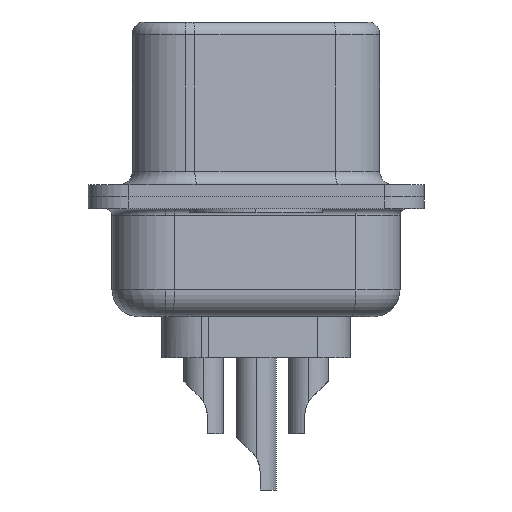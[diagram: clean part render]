
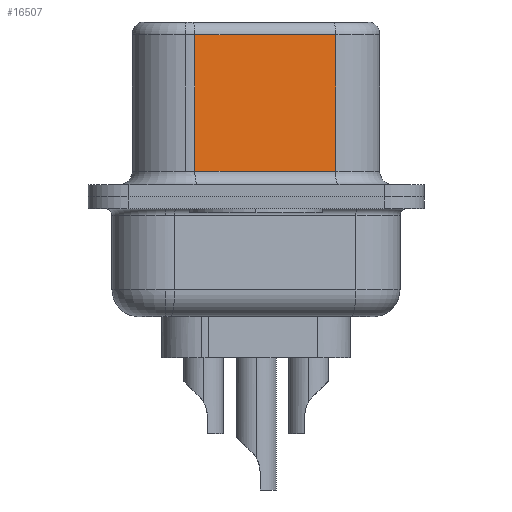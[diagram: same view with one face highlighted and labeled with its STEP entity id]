
A CAD part, left-side view. The second image highlights one B-rep face of the part: STEP entity #16507.
In plain terms, the highlighted planar face has unit normal (-0.985, -0.174, 0).
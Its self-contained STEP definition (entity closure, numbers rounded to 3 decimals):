
#114 = DIRECTION ( 'NONE',  ( 0.985, 0.174, 0. ) ) ;
#605 = AXIS2_PLACEMENT_3D ( 'NONE', #13615, #114, #6886 ) ;
#1088 = ORIENTED_EDGE ( 'NONE', *, *, #12718, .T. ) ;
#1789 = VERTEX_POINT ( 'NONE', #17715 ) ;
#2067 = LINE ( 'NONE', #8825, #8016 ) ;
#2081 = EDGE_CURVE ( 'NONE', #20152, #1789, #10763, .T. ) ;
#2378 = CARTESIAN_POINT ( 'NONE',  ( 4.546, -2.987, 0.95 ) ) ;
#2436 = ORIENTED_EDGE ( 'NONE', *, *, #13427, .F. ) ;
#3622 = DIRECTION ( 'NONE',  ( 0., 0., -1. ) ) ;
#3859 = ORIENTED_EDGE ( 'NONE', *, *, #2081, .T. ) ;
#4138 = CARTESIAN_POINT ( 'NONE',  ( 4.546, -2.987, 6.07 ) ) ;
#4976 = CARTESIAN_POINT ( 'NONE',  ( 4.546, -2.987, 0.95 ) ) ;
#5349 = DIRECTION ( 'NONE',  ( -0.174, 0.985, 0. ) ) ;
#5482 = DIRECTION ( 'NONE',  ( 0., 0., -1. ) ) ;
#6273 = VERTEX_POINT ( 'NONE', #13761 ) ;
#6886 = DIRECTION ( 'NONE',  ( -0.174, 0.985, 0. ) ) ;
#7346 = CARTESIAN_POINT ( 'NONE',  ( 4.546, -2.987, 6.07 ) ) ;
#8016 = VECTOR ( 'NONE', #3622, 1000. ) ;
#8825 = CARTESIAN_POINT ( 'NONE',  ( 3.615, 2.293, 6.57 ) ) ;
#9339 = CARTESIAN_POINT ( 'NONE',  ( 4.546, -2.987, 6.57 ) ) ;
#9367 = EDGE_LOOP ( 'NONE', ( #2436, #3859, #1088, #20185 ) ) ;
#10199 = FACE_OUTER_BOUND ( 'NONE', #9367, .T. ) ;
#10763 = LINE ( 'NONE', #7346, #10787 ) ;
#10787 = VECTOR ( 'NONE', #5349, 1000. ) ;
#10822 = DIRECTION ( 'NONE',  ( 0.174, -0.985, 0. ) ) ;
#12718 = EDGE_CURVE ( 'NONE', #1789, #6273, #2067, .T. ) ;
#13427 = EDGE_CURVE ( 'NONE', #20152, #19004, #21044, .T. ) ;
#13615 = CARTESIAN_POINT ( 'NONE',  ( 4.546, -2.987, 6.57 ) ) ;
#13761 = CARTESIAN_POINT ( 'NONE',  ( 3.615, 2.293, 0.95 ) ) ;
#16497 = VECTOR ( 'NONE', #10822, 1000. ) ;
#16507 = ADVANCED_FACE ( 'NONE', ( #10199 ), #20249, .F. ) ;
#17049 = EDGE_CURVE ( 'NONE', #6273, #19004, #20120, .T. ) ;
#17715 = CARTESIAN_POINT ( 'NONE',  ( 3.615, 2.293, 6.07 ) ) ;
#18142 = VECTOR ( 'NONE', #5482, 1000. ) ;
#19004 = VERTEX_POINT ( 'NONE', #2378 ) ;
#20120 = LINE ( 'NONE', #4976, #16497 ) ;
#20152 = VERTEX_POINT ( 'NONE', #4138 ) ;
#20185 = ORIENTED_EDGE ( 'NONE', *, *, #17049, .T. ) ;
#20249 = PLANE ( 'NONE',  #605 ) ;
#21044 = LINE ( 'NONE', #9339, #18142 ) ;
